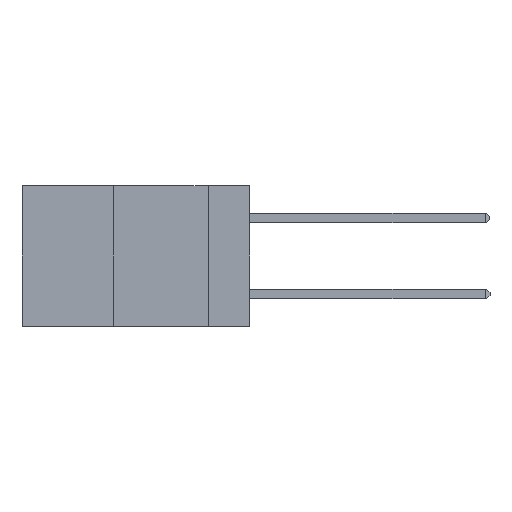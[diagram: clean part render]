
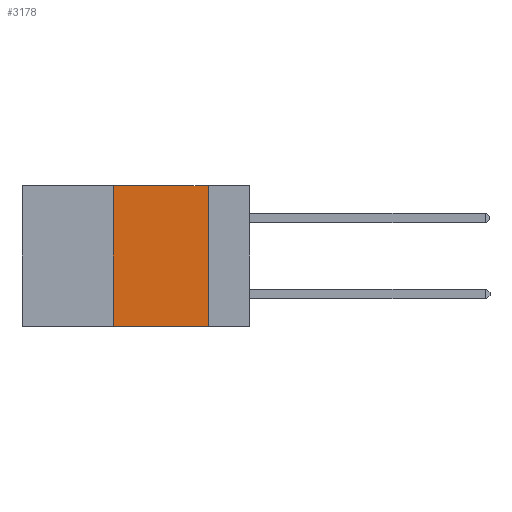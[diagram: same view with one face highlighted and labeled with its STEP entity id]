
A CAD part, left-side view. The second image highlights one B-rep face of the part: STEP entity #3178.
In plain terms, the highlighted planar face has unit normal (-1, 0, 0).
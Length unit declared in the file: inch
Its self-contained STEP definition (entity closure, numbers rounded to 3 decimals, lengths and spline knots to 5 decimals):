
#1095 = LINE ( 'NONE', #6042, #8920 ) ;
#1249 = EDGE_LOOP ( 'NONE', ( #12105, #7650, #2747, #10720 ) ) ;
#1911 = VECTOR ( 'NONE', #5230, 39.37008 ) ;
#2191 = VERTEX_POINT ( 'NONE', #10618 ) ;
#2642 = VERTEX_POINT ( 'NONE', #3856 ) ;
#2747 = ORIENTED_EDGE ( 'NONE', *, *, #3174, .F. ) ;
#2864 = VERTEX_POINT ( 'NONE', #10475 ) ;
#3171 = EDGE_CURVE ( 'NONE', #11547, #2642, #12231, .T. ) ;
#3174 = EDGE_CURVE ( 'NONE', #2191, #2864, #11962, .T. ) ;
#3178 = ADVANCED_FACE ( 'NONE', ( #9354 ), #5092, .F. ) ;
#3856 = CARTESIAN_POINT ( 'NONE',  ( 0., 0.11, -0.37 ) ) ;
#4313 = EDGE_CURVE ( 'NONE', #2191, #2642, #1095, .T. ) ;
#5004 = DIRECTION ( 'NONE',  ( 0., 0., -1. ) ) ;
#5092 = PLANE ( 'NONE',  #7386 ) ;
#5093 = DIRECTION ( 'NONE',  ( 1., 0., 0. ) ) ;
#5188 = CARTESIAN_POINT ( 'NONE',  ( 0., 0.6, 0. ) ) ;
#5230 = DIRECTION ( 'NONE',  ( 0., 0., 1. ) ) ;
#5313 = CARTESIAN_POINT ( 'NONE',  ( 0., 0.36, 0. ) ) ;
#5478 = CARTESIAN_POINT ( 'NONE',  ( 0., 0.11, 0. ) ) ;
#5495 = DIRECTION ( 'NONE',  ( 0., 0., -1. ) ) ;
#5996 = CARTESIAN_POINT ( 'NONE',  ( 0., 0.11, 0. ) ) ;
#6020 = DIRECTION ( 'NONE',  ( 0., -1., 0. ) ) ;
#6042 = CARTESIAN_POINT ( 'NONE',  ( 0., 0.6, -0.37 ) ) ;
#6176 = DIRECTION ( 'NONE',  ( 0., -1., 0. ) ) ;
#7386 = AXIS2_PLACEMENT_3D ( 'NONE', #5188, #5093, #5004 ) ;
#7492 = VECTOR ( 'NONE', #5495, 39.37008 ) ;
#7650 = ORIENTED_EDGE ( 'NONE', *, *, #10715, .F. ) ;
#8148 = VECTOR ( 'NONE', #6176, 39.37008 ) ;
#8920 = VECTOR ( 'NONE', #6020, 39.37008 ) ;
#9354 = FACE_OUTER_BOUND ( 'NONE', #1249, .T. ) ;
#9779 = CARTESIAN_POINT ( 'NONE',  ( 0., 0.6, 0. ) ) ;
#10475 = CARTESIAN_POINT ( 'NONE',  ( 0., 0.36, 0. ) ) ;
#10559 = LINE ( 'NONE', #9779, #8148 ) ;
#10618 = CARTESIAN_POINT ( 'NONE',  ( 0., 0.36, -0.37 ) ) ;
#10715 = EDGE_CURVE ( 'NONE', #2864, #11547, #10559, .T. ) ;
#10720 = ORIENTED_EDGE ( 'NONE', *, *, #4313, .T. ) ;
#11547 = VERTEX_POINT ( 'NONE', #5996 ) ;
#11962 = LINE ( 'NONE', #5313, #1911 ) ;
#12105 = ORIENTED_EDGE ( 'NONE', *, *, #3171, .F. ) ;
#12231 = LINE ( 'NONE', #5478, #7492 ) ;
